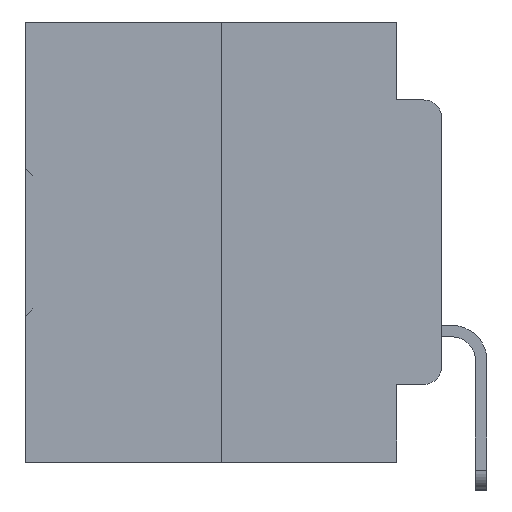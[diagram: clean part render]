
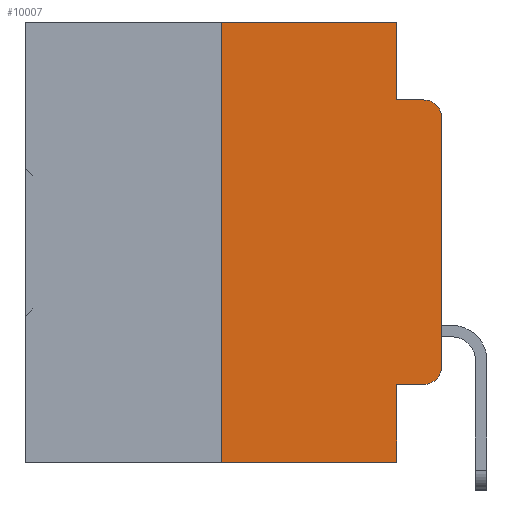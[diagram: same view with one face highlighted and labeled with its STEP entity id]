
A CAD part, left-side view. The second image highlights one B-rep face of the part: STEP entity #10007.
In plain terms, the highlighted planar face has unit normal (-1, 0, 0).
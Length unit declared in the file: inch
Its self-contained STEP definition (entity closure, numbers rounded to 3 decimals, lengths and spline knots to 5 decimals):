
#637 = DIRECTION ( 'NONE',  ( 0., -1., 0. ) ) ;
#1259 = LINE ( 'NONE', #19220, #8718 ) ;
#1290 = AXIS2_PLACEMENT_3D ( 'NONE', #16151, #13540, #32265 ) ;
#3684 = CIRCLE ( 'NONE', #27467, 0.02 ) ;
#4539 = DIRECTION ( 'NONE',  ( -1., 0., 0. ) ) ;
#4871 = VERTEX_POINT ( 'NONE', #29742 ) ;
#5216 = DIRECTION ( 'NONE',  ( 0., -1., 0. ) ) ;
#5504 = DIRECTION ( 'NONE',  ( 0., 0., 1. ) ) ;
#6124 = EDGE_CURVE ( 'NONE', #18563, #24347, #26355, .T. ) ;
#6407 = LINE ( 'NONE', #20433, #20120 ) ;
#7135 = VECTOR ( 'NONE', #5216, 39.37008 ) ;
#7159 = VERTEX_POINT ( 'NONE', #23830 ) ;
#7198 = ORIENTED_EDGE ( 'NONE', *, *, #18834, .F. ) ;
#7353 = LINE ( 'NONE', #19405, #21022 ) ;
#7661 = ORIENTED_EDGE ( 'NONE', *, *, #22845, .T. ) ;
#8022 = EDGE_CURVE ( 'NONE', #18404, #7159, #27876, .T. ) ;
#8594 = CARTESIAN_POINT ( 'NONE',  ( 0., 0.051, 0. ) ) ;
#8718 = VECTOR ( 'NONE', #5504, 39.37008 ) ;
#9586 = DIRECTION ( 'NONE',  ( 0., 0., -1. ) ) ;
#10007 = ADVANCED_FACE ( 'NONE', ( #23573 ), #10757, .F. ) ;
#10757 = PLANE ( 'NONE',  #1290 ) ;
#12420 = CARTESIAN_POINT ( 'NONE',  ( 0., 0.051, 0. ) ) ;
#13099 = EDGE_CURVE ( 'NONE', #16760, #34248, #3684, .T. ) ;
#13540 = DIRECTION ( 'NONE',  ( 1., 0., 0. ) ) ;
#14205 = CARTESIAN_POINT ( 'NONE',  ( 0., 0.051, -0.4115 ) ) ;
#14308 = LINE ( 'NONE', #33197, #27750 ) ;
#14900 = CARTESIAN_POINT ( 'NONE',  ( 0., 0.02, -0.4115 ) ) ;
#15483 = CARTESIAN_POINT ( 'NONE',  ( 0., 0.02, -0.3915 ) ) ;
#15767 = VECTOR ( 'NONE', #29543, 39.37008 ) ;
#15874 = EDGE_CURVE ( 'NONE', #30250, #33570, #14308, .T. ) ;
#16151 = CARTESIAN_POINT ( 'NONE',  ( 0., 0.473, 0. ) ) ;
#16163 = EDGE_LOOP ( 'NONE', ( #17901, #20439, #22982, #25482, #26292, #7198, #30460, #28393, #7661, #30877 ) ) ;
#16227 = LINE ( 'NONE', #12420, #29604 ) ;
#16674 = DIRECTION ( 'NONE',  ( 0., -1., 0. ) ) ;
#16760 = VERTEX_POINT ( 'NONE', #14900 ) ;
#16828 = CARTESIAN_POINT ( 'NONE',  ( 0., 0.473, 0. ) ) ;
#17420 = EDGE_CURVE ( 'NONE', #22406, #33570, #6407, .T. ) ;
#17901 = ORIENTED_EDGE ( 'NONE', *, *, #21285, .T. ) ;
#18237 = DIRECTION ( 'NONE',  ( 0., 0., -1. ) ) ;
#18404 = VERTEX_POINT ( 'NONE', #27264 ) ;
#18563 = VERTEX_POINT ( 'NONE', #27843 ) ;
#18619 = EDGE_CURVE ( 'NONE', #24347, #4871, #16227, .T. ) ;
#18834 = EDGE_CURVE ( 'NONE', #30250, #18563, #22966, .T. ) ;
#18861 = CARTESIAN_POINT ( 'NONE',  ( 0., 0.25, -0.5 ) ) ;
#19220 = CARTESIAN_POINT ( 'NONE',  ( 0., 0., 0. ) ) ;
#19405 = CARTESIAN_POINT ( 'NONE',  ( 0., 0.051, -0.0885 ) ) ;
#20120 = VECTOR ( 'NONE', #9586, 39.37008 ) ;
#20433 = CARTESIAN_POINT ( 'NONE',  ( 0., 0.051, 0. ) ) ;
#20439 = ORIENTED_EDGE ( 'NONE', *, *, #8022, .T. ) ;
#20975 = CARTESIAN_POINT ( 'NONE',  ( 0., 0.02, -0.1085 ) ) ;
#21022 = VECTOR ( 'NONE', #16674, 39.37008 ) ;
#21285 = EDGE_CURVE ( 'NONE', #34248, #18404, #1259, .T. ) ;
#21963 = EDGE_CURVE ( 'NONE', #4871, #7159, #7353, .T. ) ;
#22406 = VERTEX_POINT ( 'NONE', #14205 ) ;
#22845 = EDGE_CURVE ( 'NONE', #22406, #16760, #28733, .T. ) ;
#22966 = LINE ( 'NONE', #34799, #15767 ) ;
#22982 = ORIENTED_EDGE ( 'NONE', *, *, #21963, .F. ) ;
#23573 = FACE_OUTER_BOUND ( 'NONE', #16163, .T. ) ;
#23698 = DIRECTION ( 'NONE',  ( 0., 0., -1. ) ) ;
#23830 = CARTESIAN_POINT ( 'NONE',  ( 0., 0.02, -0.0885 ) ) ;
#24347 = VERTEX_POINT ( 'NONE', #8594 ) ;
#24716 = VECTOR ( 'NONE', #32935, 39.37008 ) ;
#25482 = ORIENTED_EDGE ( 'NONE', *, *, #18619, .F. ) ;
#25857 = DIRECTION ( 'NONE',  ( 0., 0., -1. ) ) ;
#26265 = CARTESIAN_POINT ( 'NONE',  ( 0., 0., -0.3915 ) ) ;
#26292 = ORIENTED_EDGE ( 'NONE', *, *, #6124, .F. ) ;
#26355 = LINE ( 'NONE', #16828, #24716 ) ;
#27264 = CARTESIAN_POINT ( 'NONE',  ( 0., 0., -0.1085 ) ) ;
#27467 = AXIS2_PLACEMENT_3D ( 'NONE', #15483, #34193, #18237 ) ;
#27750 = VECTOR ( 'NONE', #637, 39.37008 ) ;
#27843 = CARTESIAN_POINT ( 'NONE',  ( 0., 0.25, 0. ) ) ;
#27876 = CIRCLE ( 'NONE', #33039, 0.02 ) ;
#28393 = ORIENTED_EDGE ( 'NONE', *, *, #17420, .F. ) ;
#28733 = LINE ( 'NONE', #34910, #7135 ) ;
#28843 = CARTESIAN_POINT ( 'NONE',  ( 0., 0.051, -0.5 ) ) ;
#29543 = DIRECTION ( 'NONE',  ( 0., 0., 1. ) ) ;
#29604 = VECTOR ( 'NONE', #25857, 39.37008 ) ;
#29742 = CARTESIAN_POINT ( 'NONE',  ( 0., 0.051, -0.0885 ) ) ;
#30250 = VERTEX_POINT ( 'NONE', #18861 ) ;
#30460 = ORIENTED_EDGE ( 'NONE', *, *, #15874, .T. ) ;
#30877 = ORIENTED_EDGE ( 'NONE', *, *, #13099, .T. ) ;
#32265 = DIRECTION ( 'NONE',  ( 0., 0., -1. ) ) ;
#32935 = DIRECTION ( 'NONE',  ( 0., -1., 0. ) ) ;
#33039 = AXIS2_PLACEMENT_3D ( 'NONE', #20975, #4539, #23698 ) ;
#33197 = CARTESIAN_POINT ( 'NONE',  ( 0., 0.473, -0.5 ) ) ;
#33570 = VERTEX_POINT ( 'NONE', #28843 ) ;
#34193 = DIRECTION ( 'NONE',  ( -1., 0., 0. ) ) ;
#34248 = VERTEX_POINT ( 'NONE', #26265 ) ;
#34799 = CARTESIAN_POINT ( 'NONE',  ( 0., 0.25, 0. ) ) ;
#34910 = CARTESIAN_POINT ( 'NONE',  ( 0., 0.051, -0.4115 ) ) ;
